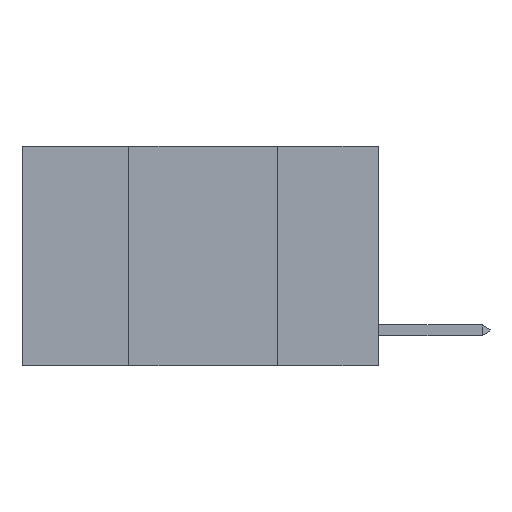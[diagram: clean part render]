
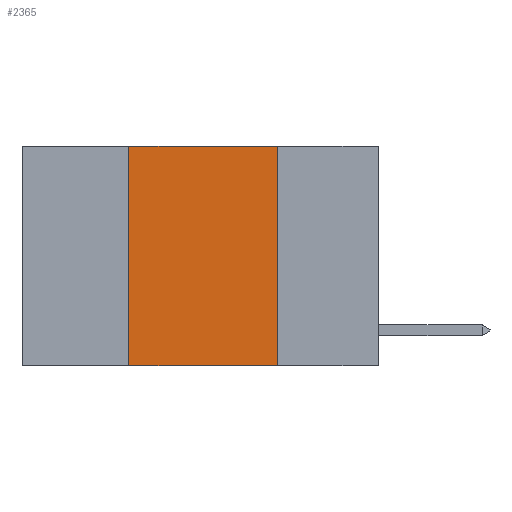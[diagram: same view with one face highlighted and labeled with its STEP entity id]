
A CAD part, left-side view. The second image highlights one B-rep face of the part: STEP entity #2365.
In plain terms, the highlighted planar face has unit normal (-1, 0, 0).
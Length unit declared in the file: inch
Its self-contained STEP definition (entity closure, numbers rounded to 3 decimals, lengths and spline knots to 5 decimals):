
#322 = VERTEX_POINT ( 'NONE', #13495 ) ;
#672 = LINE ( 'NONE', #19519, #18623 ) ;
#991 = EDGE_CURVE ( 'NONE', #17265, #9129, #4047, .T. ) ;
#1475 = DIRECTION ( 'NONE',  ( 1., 0., 0. ) ) ;
#2365 = ADVANCED_FACE ( 'NONE', ( #3126 ), #15262, .F. ) ;
#2592 = LINE ( 'NONE', #13016, #20474 ) ;
#3036 = DIRECTION ( 'NONE',  ( 0., 0., 1. ) ) ;
#3126 = FACE_OUTER_BOUND ( 'NONE', #21918, .T. ) ;
#4047 = LINE ( 'NONE', #11130, #8122 ) ;
#7665 = CARTESIAN_POINT ( 'NONE',  ( 0., 0.42, 0. ) ) ;
#7911 = EDGE_CURVE ( 'NONE', #9129, #17249, #18826, .T. ) ;
#8024 = ORIENTED_EDGE ( 'NONE', *, *, #14551, .T. ) ;
#8122 = VECTOR ( 'NONE', #3036, 39.37008 ) ;
#9129 = VERTEX_POINT ( 'NONE', #7665 ) ;
#9481 = CARTESIAN_POINT ( 'NONE',  ( 0., 0.6, 0. ) ) ;
#10643 = AXIS2_PLACEMENT_3D ( 'NONE', #22182, #1475, #13654 ) ;
#11130 = CARTESIAN_POINT ( 'NONE',  ( 0., 0.42, 0. ) ) ;
#11237 = DIRECTION ( 'NONE',  ( 0., -1., 0. ) ) ;
#13016 = CARTESIAN_POINT ( 'NONE',  ( 0., 0.6, -0.37 ) ) ;
#13495 = CARTESIAN_POINT ( 'NONE',  ( 0., 0.17, -0.37 ) ) ;
#13527 = CARTESIAN_POINT ( 'NONE',  ( 0., 0.17, 0. ) ) ;
#13654 = DIRECTION ( 'NONE',  ( 0., 0., -1. ) ) ;
#14399 = EDGE_CURVE ( 'NONE', #17249, #322, #672, .T. ) ;
#14551 = EDGE_CURVE ( 'NONE', #17265, #322, #2592, .T. ) ;
#14903 = ORIENTED_EDGE ( 'NONE', *, *, #14399, .F. ) ;
#15164 = ORIENTED_EDGE ( 'NONE', *, *, #991, .F. ) ;
#15262 = PLANE ( 'NONE',  #10643 ) ;
#15457 = ORIENTED_EDGE ( 'NONE', *, *, #7911, .F. ) ;
#17249 = VERTEX_POINT ( 'NONE', #13527 ) ;
#17265 = VERTEX_POINT ( 'NONE', #18731 ) ;
#17899 = DIRECTION ( 'NONE',  ( 0., 0., -1. ) ) ;
#18623 = VECTOR ( 'NONE', #17899, 39.37008 ) ;
#18731 = CARTESIAN_POINT ( 'NONE',  ( 0., 0.42, -0.37 ) ) ;
#18826 = LINE ( 'NONE', #9481, #19363 ) ;
#19363 = VECTOR ( 'NONE', #11237, 39.37008 ) ;
#19519 = CARTESIAN_POINT ( 'NONE',  ( 0., 0.17, 0. ) ) ;
#19957 = DIRECTION ( 'NONE',  ( 0., -1., 0. ) ) ;
#20474 = VECTOR ( 'NONE', #19957, 39.37008 ) ;
#21918 = EDGE_LOOP ( 'NONE', ( #14903, #15457, #15164, #8024 ) ) ;
#22182 = CARTESIAN_POINT ( 'NONE',  ( 0., 0.6, 0. ) ) ;
